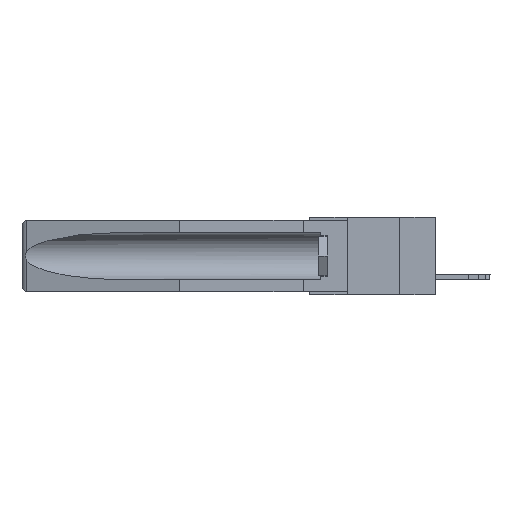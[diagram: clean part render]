
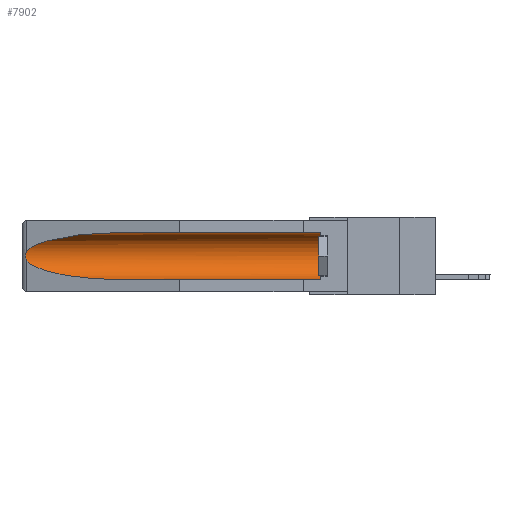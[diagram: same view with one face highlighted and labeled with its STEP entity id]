
A CAD part, left-side view. The second image highlights one B-rep face of the part: STEP entity #7902.
In plain terms, the highlighted cylindrical face has radius 2.857 mm (diameter 5.715 mm), a partial arc.
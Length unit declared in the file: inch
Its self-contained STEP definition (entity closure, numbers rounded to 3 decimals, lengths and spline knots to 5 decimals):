
#1340 = VERTEX_POINT ( 'NONE', #2041 ) ;
#1846 = CARTESIAN_POINT ( 'NONE',  ( 0.25451, 1.48313, -0.09465 ) ) ;
#1906 = CARTESIAN_POINT ( 'NONE',  ( 0.2675, 1.53308, -0.17534 ) ) ;
#2041 = CARTESIAN_POINT ( 'NONE',  ( 0.155, 0.126, -0.284 ) ) ;
#3029 = ORIENTED_EDGE ( 'NONE', *, *, #28066, .T. ) ;
#3968 = CARTESIAN_POINT ( 'NONE',  ( 0.26597, 1.52961, -0.15275 ) ) ;
#5091 = ORIENTED_EDGE ( 'NONE', *, *, #18664, .T. ) ;
#5128 = CARTESIAN_POINT ( 'NONE',  ( 0.155, 0.126, -0.1715 ) ) ;
#5589 = ORIENTED_EDGE ( 'NONE', *, *, #8473, .T. ) ;
#6412 = DIRECTION ( 'NONE',  ( 0., 1., 0. ) ) ;
#6444 = VERTEX_POINT ( 'NONE', #28059 ) ;
#6487 = VERTEX_POINT ( 'NONE', #23831 ) ;
#7902 = ADVANCED_FACE ( 'NONE', ( #10226 ), #27633, .F. ) ;
#8020 = CARTESIAN_POINT ( 'NONE',  ( 0.155, 1.07973, -0.059 ) ) ;
#8125 = EDGE_CURVE ( 'NONE', #17243, #6444, #21025, .T. ) ;
#8473 = EDGE_CURVE ( 'NONE', #8680, #17243, #15949, .T. ) ;
#8552 = CARTESIAN_POINT ( 'NONE',  ( 0.2673, 1.5327, -0.16383 ) ) ;
#8680 = VERTEX_POINT ( 'NONE', #26121 ) ;
#8942 = CIRCLE ( 'NONE', #24216, 0.1125 ) ;
#9081 = CARTESIAN_POINT ( 'NONE',  ( 0.155, -0.30754, -0.1715 ) ) ;
#9232 = EDGE_LOOP ( 'NONE', ( #20492, #5091, #25791, #18014, #3029, #5589 ) ) ;
#10226 = FACE_OUTER_BOUND ( 'NONE', #9232, .T. ) ;
#10315 = CARTESIAN_POINT ( 'NONE',  ( 0.26537, 1.52718, -0.14972 ) ) ;
#11139 = CARTESIAN_POINT ( 'NONE',  ( 0.155, 1.07973, -0.284 ) ) ;
#11710 = CARTESIAN_POINT ( 'NONE',  ( 0.155, 1.07973, -0.284 ) ) ;
#12626 = CARTESIAN_POINT ( 'NONE',  ( 0.155, 1.07973, -0.059 ) ) ;
#12959 = CARTESIAN_POINT ( 'NONE',  ( 0.155, -0.30754, -0.059 ) ) ;
#13889 = VERTEX_POINT ( 'NONE', #11139 ) ;
#13973 = DIRECTION ( 'NONE',  ( 0., 0., 1. ) ) ;
#14451 = CARTESIAN_POINT ( 'NONE',  ( 0.26537, 1.52718, -0.14972 ) ) ;
#15949 = LINE ( 'NONE', #12959, #20409 ) ;
#16049 = DIRECTION ( 'NONE',  ( 0., -1., 0. ) ) ;
#17201 = LINE ( 'NONE', #20345, #20587 ) ;
#17243 = VERTEX_POINT ( 'NONE', #8020 ) ;
#17521 = DIRECTION ( 'NONE',  ( 0., 1., 0. ) ) ;
#18014 = ORIENTED_EDGE ( 'NONE', *, *, #24392, .F. ) ;
#18220 = B_SPLINE_CURVE_WITH_KNOTS ( 'NONE', 3,
 ( #10315, #3968, #25762, #8552, #21164, #1906, #23746, #23463, #19153, #25566 ),
 .UNSPECIFIED., .F., .F.,
 ( 4, 2, 2, 2, 4 ),
 ( 0., 0.00029, 0.00058, 0.00087, 0.00117 ),
 .UNSPECIFIED. ) ;
#18664 = EDGE_CURVE ( 'NONE', #6444, #6487, #18220, .T. ) ;
#18734 =( BOUNDED_CURVE ( )  B_SPLINE_CURVE ( 3, ( #20077, #22449, #22659, #11710 ),
 .UNSPECIFIED., .F., .F. ) 
 B_SPLINE_CURVE_WITH_KNOTS ( ( 4, 4 ),
 ( 0.1948, 1.5708 ),
 .UNSPECIFIED. ) 
 CURVE ( )  GEOMETRIC_REPRESENTATION_ITEM ( )  RATIONAL_B_SPLINE_CURVE ( ( 1., 0.848, 0.848, 1. ) ) 
 REPRESENTATION_ITEM ( '' )  );
#19153 = CARTESIAN_POINT ( 'NONE',  ( 0.26597, 1.5296, -0.19026 ) ) ;
#19486 = AXIS2_PLACEMENT_3D ( 'NONE', #9081, #17521, #19904 ) ;
#19608 = EDGE_CURVE ( 'NONE', #6487, #13889, #18734, .T. ) ;
#19904 = DIRECTION ( 'NONE',  ( 0., 0., 1. ) ) ;
#20077 = CARTESIAN_POINT ( 'NONE',  ( 0.26537, 1.52718, -0.19328 ) ) ;
#20345 = CARTESIAN_POINT ( 'NONE',  ( 0.155, -0.30754, -0.284 ) ) ;
#20409 = VECTOR ( 'NONE', #6412, 39.37008 ) ;
#20492 = ORIENTED_EDGE ( 'NONE', *, *, #8125, .T. ) ;
#20587 = VECTOR ( 'NONE', #22806, 39.37008 ) ;
#21025 =( BOUNDED_CURVE ( )  B_SPLINE_CURVE ( 3, ( #12626, #27905, #1846, #14451 ),
 .UNSPECIFIED., .F., .F. ) 
 B_SPLINE_CURVE_WITH_KNOTS ( ( 4, 4 ),
 ( 4.71239, 6.08839 ),
 .UNSPECIFIED. ) 
 CURVE ( )  GEOMETRIC_REPRESENTATION_ITEM ( )  RATIONAL_B_SPLINE_CURVE ( ( 1., 0.848, 0.848, 1. ) ) 
 REPRESENTATION_ITEM ( '' )  );
#21164 = CARTESIAN_POINT ( 'NONE',  ( 0.2675, 1.53308, -0.16763 ) ) ;
#22449 = CARTESIAN_POINT ( 'NONE',  ( 0.25451, 1.48313, -0.24835 ) ) ;
#22659 = CARTESIAN_POINT ( 'NONE',  ( 0.21114, 1.30732, -0.284 ) ) ;
#22806 = DIRECTION ( 'NONE',  ( 0., 1., 0. ) ) ;
#23463 = CARTESIAN_POINT ( 'NONE',  ( 0.26655, 1.53094, -0.18657 ) ) ;
#23746 = CARTESIAN_POINT ( 'NONE',  ( 0.2673, 1.53269, -0.17917 ) ) ;
#23831 = CARTESIAN_POINT ( 'NONE',  ( 0.26537, 1.52718, -0.19328 ) ) ;
#24216 = AXIS2_PLACEMENT_3D ( 'NONE', #5128, #16049, #13973 ) ;
#24392 = EDGE_CURVE ( 'NONE', #1340, #13889, #17201, .T. ) ;
#25566 = CARTESIAN_POINT ( 'NONE',  ( 0.26537, 1.52718, -0.19328 ) ) ;
#25762 = CARTESIAN_POINT ( 'NONE',  ( 0.26654, 1.53092, -0.15636 ) ) ;
#25791 = ORIENTED_EDGE ( 'NONE', *, *, #19608, .T. ) ;
#26121 = CARTESIAN_POINT ( 'NONE',  ( 0.155, 0.126, -0.059 ) ) ;
#27633 = CYLINDRICAL_SURFACE ( 'NONE', #19486, 0.1125 ) ;
#27905 = CARTESIAN_POINT ( 'NONE',  ( 0.21114, 1.30732, -0.059 ) ) ;
#28059 = CARTESIAN_POINT ( 'NONE',  ( 0.26537, 1.52718, -0.14972 ) ) ;
#28066 = EDGE_CURVE ( 'NONE', #1340, #8680, #8942, .T. ) ;
